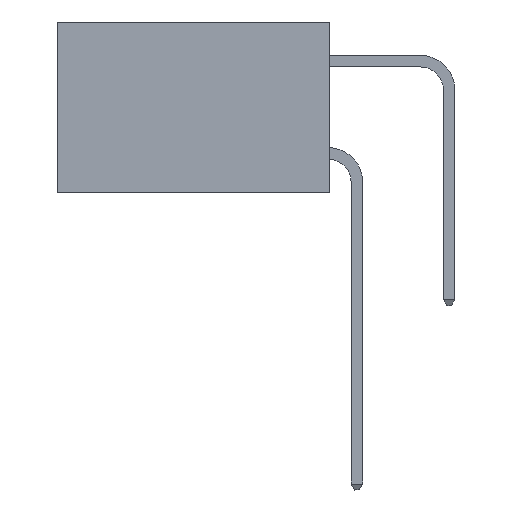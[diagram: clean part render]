
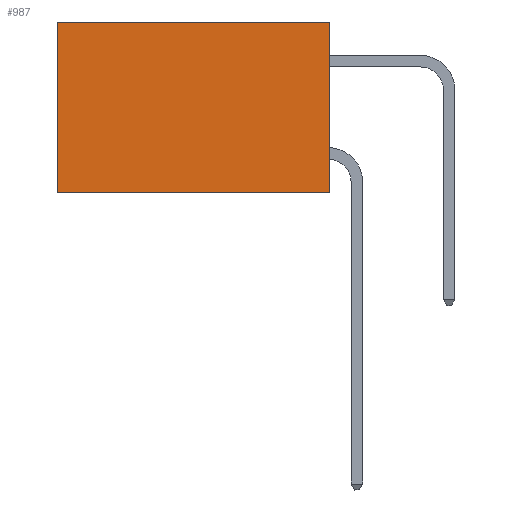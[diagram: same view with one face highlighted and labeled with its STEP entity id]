
A CAD part, left-side view. The second image highlights one B-rep face of the part: STEP entity #987.
In plain terms, the highlighted planar face has unit normal (-1, 0, 0).
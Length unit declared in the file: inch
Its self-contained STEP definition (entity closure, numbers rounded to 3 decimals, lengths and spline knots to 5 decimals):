
#940 = VERTEX_POINT ( 'NONE', #14417 ) ;
#987 = ADVANCED_FACE ( 'NONE', ( #30959 ), #8650, .F. ) ;
#1449 = LINE ( 'NONE', #23117, #20563 ) ;
#1992 = VERTEX_POINT ( 'NONE', #8500 ) ;
#2244 = VECTOR ( 'NONE', #19960, 39.37008 ) ;
#3045 = LINE ( 'NONE', #19862, #2244 ) ;
#3671 = ORIENTED_EDGE ( 'NONE', *, *, #26626, .F. ) ;
#4549 = CARTESIAN_POINT ( 'NONE',  ( 0.277, 0., 0. ) ) ;
#5352 = VECTOR ( 'NONE', #18951, 39.37008 ) ;
#5713 = ORIENTED_EDGE ( 'NONE', *, *, #13270, .T. ) ;
#7007 = CARTESIAN_POINT ( 'NONE',  ( 0.277, 0.59, -0.37 ) ) ;
#8499 = EDGE_CURVE ( 'NONE', #30666, #940, #3045, .T. ) ;
#8500 = CARTESIAN_POINT ( 'NONE',  ( 0.277, 0., -0.37 ) ) ;
#8650 = PLANE ( 'NONE',  #17720 ) ;
#8952 = ORIENTED_EDGE ( 'NONE', *, *, #8499, .T. ) ;
#9184 = ORIENTED_EDGE ( 'NONE', *, *, #9780, .F. ) ;
#9189 = VERTEX_POINT ( 'NONE', #7007 ) ;
#9780 = EDGE_CURVE ( 'NONE', #30666, #1992, #24307, .T. ) ;
#10037 = VECTOR ( 'NONE', #23152, 39.37008 ) ;
#10305 = DIRECTION ( 'NONE',  ( 0., 0., -1. ) ) ;
#10371 = DIRECTION ( 'NONE',  ( 1., 0., 0. ) ) ;
#10430 = CARTESIAN_POINT ( 'NONE',  ( 0.277, 0., -0.37 ) ) ;
#10816 = CARTESIAN_POINT ( 'NONE',  ( 0.277, 0.59, -0.37 ) ) ;
#13270 = EDGE_CURVE ( 'NONE', #940, #9189, #23985, .T. ) ;
#14417 = CARTESIAN_POINT ( 'NONE',  ( 0.277, 0.59, 0. ) ) ;
#16375 = CARTESIAN_POINT ( 'NONE',  ( 0.277, 0., -0.37 ) ) ;
#17720 = AXIS2_PLACEMENT_3D ( 'NONE', #10430, #10371, #10305 ) ;
#18951 = DIRECTION ( 'NONE',  ( 0., 0., -1. ) ) ;
#19862 = CARTESIAN_POINT ( 'NONE',  ( 0.277, 0., 0. ) ) ;
#19960 = DIRECTION ( 'NONE',  ( 0., 1., 0. ) ) ;
#20563 = VECTOR ( 'NONE', #25546, 39.37008 ) ;
#23117 = CARTESIAN_POINT ( 'NONE',  ( 0.277, 0., -0.37 ) ) ;
#23152 = DIRECTION ( 'NONE',  ( 0., 0., -1. ) ) ;
#23985 = LINE ( 'NONE', #10816, #10037 ) ;
#24307 = LINE ( 'NONE', #16375, #5352 ) ;
#25546 = DIRECTION ( 'NONE',  ( 0., 1., 0. ) ) ;
#26626 = EDGE_CURVE ( 'NONE', #1992, #9189, #1449, .T. ) ;
#29677 = EDGE_LOOP ( 'NONE', ( #5713, #3671, #9184, #8952 ) ) ;
#30666 = VERTEX_POINT ( 'NONE', #4549 ) ;
#30959 = FACE_OUTER_BOUND ( 'NONE', #29677, .T. ) ;
